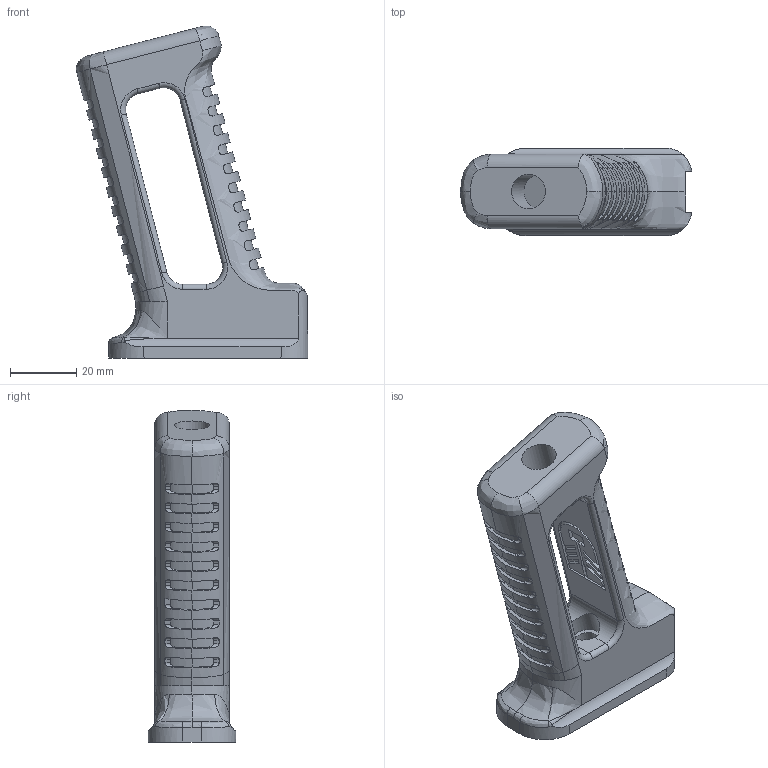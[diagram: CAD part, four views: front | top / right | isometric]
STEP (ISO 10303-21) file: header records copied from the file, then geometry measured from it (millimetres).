
FILE_DESCRIPTION(/* description */ (''),/* implementation_level */ '2;1');
FILE_NAME(/* name */ 'AK Grip Custom Skeletonized Final.step',/* time_stamp */ '2022-04-29T19:34:09-05:00',/* author */ (''),/* organization */ (''),/* preprocessor_version */ 'ST-DEVELOPER v18.1',/* originating_system */ 'Autodesk Translation Framework v10.14.0.1471',/* authorisation */ '');
FILE_SCHEMA (('AUTOMOTIVE_DESIGN { 1 0 10303 214 3 1 1 }'));
Length unit declared in the file: millimetre
Products named in the file (1): AK Grip Custom Skeletonized
Bounding box: 69.69 x 26.5 x 100.06 mm (x, y, z)
Volume: 55413.7 mm3; surface area: 17657.3 mm2
Topology: 1 solids, 1 shells, 365 faces, 1038 edges, 673 vertices
Faces by surface type: plane 177, cylinder 106, bspline 74, torus 8
Full cylindrical faces by diameter (mm): 8 x1, 10.5 x2
Entity records: 27990 total; most frequent: CARTESIAN_POINT 19533, ORIENTED_EDGE 2070, DIRECTION 1244, EDGE_CURVE 1035, VERTEX_POINT 673, LINE 520, VECTOR 520, B_SPLINE_CURVE_WITH_KNOTS 445
